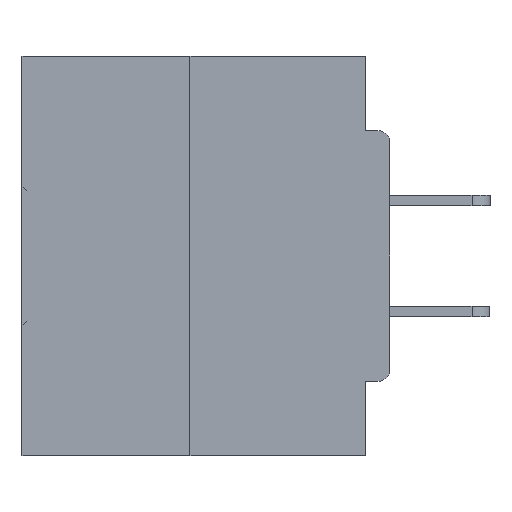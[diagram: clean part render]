
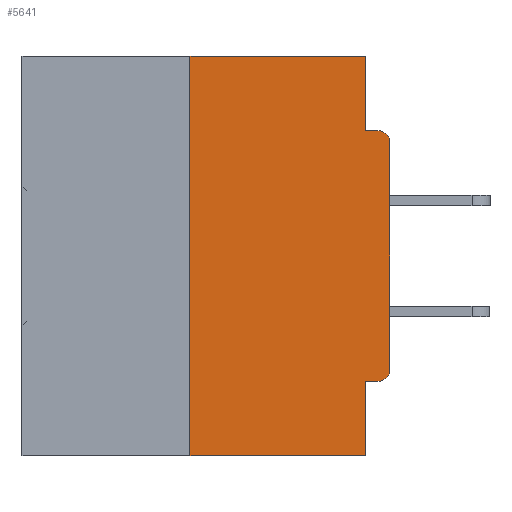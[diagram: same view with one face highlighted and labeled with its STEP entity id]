
A CAD part, left-side view. The second image highlights one B-rep face of the part: STEP entity #5641.
In plain terms, the highlighted planar face has unit normal (-1, 0, 0).
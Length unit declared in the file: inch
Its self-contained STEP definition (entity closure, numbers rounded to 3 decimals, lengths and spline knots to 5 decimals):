
#366 = AXIS2_PLACEMENT_3D ( 'NONE', #17721, #7560, #28203 ) ;
#1079 = DIRECTION ( 'NONE',  ( 0., 0., -1. ) ) ;
#1444 = CARTESIAN_POINT ( 'NONE',  ( 0., 0.031, -0.0935 ) ) ;
#3181 = CIRCLE ( 'NONE', #7344, 0.015 ) ;
#3258 = ORIENTED_EDGE ( 'NONE', *, *, #4106, .F. ) ;
#3412 = VECTOR ( 'NONE', #14868, 39.37008 ) ;
#3725 = LINE ( 'NONE', #20913, #28000 ) ;
#4106 = EDGE_CURVE ( 'NONE', #12967, #27052, #3725, .T. ) ;
#4382 = CARTESIAN_POINT ( 'NONE',  ( 0., 0.031, 0. ) ) ;
#5415 = VECTOR ( 'NONE', #24039, 39.37008 ) ;
#5618 = LINE ( 'NONE', #27364, #21851 ) ;
#5641 = ADVANCED_FACE ( 'NONE', ( #35970 ), #13357, .F. ) ;
#6293 = LINE ( 'NONE', #31373, #7930 ) ;
#6305 = VECTOR ( 'NONE', #1079, 39.37008 ) ;
#6513 = CARTESIAN_POINT ( 'NONE',  ( 0., 0., -0.4065 ) ) ;
#7344 = AXIS2_PLACEMENT_3D ( 'NONE', #7868, #38859, #18008 ) ;
#7560 = DIRECTION ( 'NONE',  ( -1., 0., 0. ) ) ;
#7868 = CARTESIAN_POINT ( 'NONE',  ( 0., 0.015, -0.1085 ) ) ;
#7930 = VECTOR ( 'NONE', #28223, 39.37008 ) ;
#8057 = VERTEX_POINT ( 'NONE', #17336 ) ;
#8436 = CARTESIAN_POINT ( 'NONE',  ( 0., 0., -0.3915 ) ) ;
#8759 = VECTOR ( 'NONE', #19306, 39.37008 ) ;
#10283 = EDGE_CURVE ( 'NONE', #19712, #36988, #21984, .T. ) ;
#11410 = ORIENTED_EDGE ( 'NONE', *, *, #23839, .F. ) ;
#11890 = CIRCLE ( 'NONE', #366, 0.015 ) ;
#12967 = VERTEX_POINT ( 'NONE', #39635 ) ;
#13223 = DIRECTION ( 'NONE',  ( 1., 0., 0. ) ) ;
#13357 = PLANE ( 'NONE',  #14992 ) ;
#13964 = DIRECTION ( 'NONE',  ( 0., 0., 1. ) ) ;
#14353 = VERTEX_POINT ( 'NONE', #8436 ) ;
#14516 = ORIENTED_EDGE ( 'NONE', *, *, #19994, .T. ) ;
#14672 = ORIENTED_EDGE ( 'NONE', *, *, #36377, .F. ) ;
#14717 = CARTESIAN_POINT ( 'NONE',  ( 0., 0., -0.0935 ) ) ;
#14868 = DIRECTION ( 'NONE',  ( 0., -1., 0. ) ) ;
#14964 = CARTESIAN_POINT ( 'NONE',  ( 0., 0.46, -0.5 ) ) ;
#14992 = AXIS2_PLACEMENT_3D ( 'NONE', #44479, #13223, #23928 ) ;
#17336 = CARTESIAN_POINT ( 'NONE',  ( 0., 0.015, -0.0935 ) ) ;
#17721 = CARTESIAN_POINT ( 'NONE',  ( 0., 0.015, -0.3915 ) ) ;
#18008 = DIRECTION ( 'NONE',  ( 0., 0., -1. ) ) ;
#19279 = EDGE_LOOP ( 'NONE', ( #24738, #14672, #36779, #3258, #37463, #14516, #21387, #23557, #11410, #34732 ) ) ;
#19306 = DIRECTION ( 'NONE',  ( 0., -1., 0. ) ) ;
#19307 = VERTEX_POINT ( 'NONE', #39608 ) ;
#19712 = VERTEX_POINT ( 'NONE', #4382 ) ;
#19994 = EDGE_CURVE ( 'NONE', #19307, #14353, #11890, .T. ) ;
#20134 = EDGE_CURVE ( 'NONE', #30142, #8057, #3181, .T. ) ;
#20913 = CARTESIAN_POINT ( 'NONE',  ( 0., 0.031, -0.5 ) ) ;
#21387 = ORIENTED_EDGE ( 'NONE', *, *, #30425, .T. ) ;
#21783 = CARTESIAN_POINT ( 'NONE',  ( 0., 0.031, 0. ) ) ;
#21851 = VECTOR ( 'NONE', #13964, 39.37008 ) ;
#21984 = LINE ( 'NONE', #21783, #6305 ) ;
#23310 = DIRECTION ( 'NONE',  ( 0., 0., -1. ) ) ;
#23557 = ORIENTED_EDGE ( 'NONE', *, *, #20134, .T. ) ;
#23831 = VERTEX_POINT ( 'NONE', #31991 ) ;
#23839 = EDGE_CURVE ( 'NONE', #36988, #8057, #27681, .T. ) ;
#23928 = DIRECTION ( 'NONE',  ( 0., 0., -1. ) ) ;
#24039 = DIRECTION ( 'NONE',  ( 0., 1., 0. ) ) ;
#24663 = EDGE_CURVE ( 'NONE', #23831, #27052, #25502, .T. ) ;
#24738 = ORIENTED_EDGE ( 'NONE', *, *, #38163, .F. ) ;
#25502 = LINE ( 'NONE', #14964, #8759 ) ;
#25532 = EDGE_CURVE ( 'NONE', #19307, #12967, #33474, .T. ) ;
#26180 = CARTESIAN_POINT ( 'NONE',  ( 0., 0., -0.1085 ) ) ;
#27052 = VERTEX_POINT ( 'NONE', #43616 ) ;
#27364 = CARTESIAN_POINT ( 'NONE',  ( 0., 0., 0. ) ) ;
#27681 = LINE ( 'NONE', #14717, #3412 ) ;
#27899 = DIRECTION ( 'NONE',  ( 0., -1., 0. ) ) ;
#28000 = VECTOR ( 'NONE', #23310, 39.37008 ) ;
#28196 = CARTESIAN_POINT ( 'NONE',  ( 0., 0.46, 0. ) ) ;
#28203 = DIRECTION ( 'NONE',  ( 0., 0., -1. ) ) ;
#28223 = DIRECTION ( 'NONE',  ( 0., 0., 1. ) ) ;
#30142 = VERTEX_POINT ( 'NONE', #26180 ) ;
#30425 = EDGE_CURVE ( 'NONE', #14353, #30142, #5618, .T. ) ;
#30764 = VERTEX_POINT ( 'NONE', #36049 ) ;
#31373 = CARTESIAN_POINT ( 'NONE',  ( 0., 0.25, 0. ) ) ;
#31991 = CARTESIAN_POINT ( 'NONE',  ( 0., 0.25, -0.5 ) ) ;
#33474 = LINE ( 'NONE', #6513, #5415 ) ;
#34732 = ORIENTED_EDGE ( 'NONE', *, *, #10283, .F. ) ;
#35970 = FACE_OUTER_BOUND ( 'NONE', #19279, .T. ) ;
#36049 = CARTESIAN_POINT ( 'NONE',  ( 0., 0.25, 0. ) ) ;
#36377 = EDGE_CURVE ( 'NONE', #23831, #30764, #6293, .T. ) ;
#36599 = VECTOR ( 'NONE', #27899, 39.37008 ) ;
#36779 = ORIENTED_EDGE ( 'NONE', *, *, #24663, .T. ) ;
#36988 = VERTEX_POINT ( 'NONE', #1444 ) ;
#37463 = ORIENTED_EDGE ( 'NONE', *, *, #25532, .F. ) ;
#38163 = EDGE_CURVE ( 'NONE', #30764, #19712, #44135, .T. ) ;
#38859 = DIRECTION ( 'NONE',  ( -1., 0., 0. ) ) ;
#39608 = CARTESIAN_POINT ( 'NONE',  ( 0., 0.015, -0.4065 ) ) ;
#39635 = CARTESIAN_POINT ( 'NONE',  ( 0., 0.031, -0.4065 ) ) ;
#43616 = CARTESIAN_POINT ( 'NONE',  ( 0., 0.031, -0.5 ) ) ;
#44135 = LINE ( 'NONE', #28196, #36599 ) ;
#44479 = CARTESIAN_POINT ( 'NONE',  ( 0., 0.46, 0. ) ) ;
